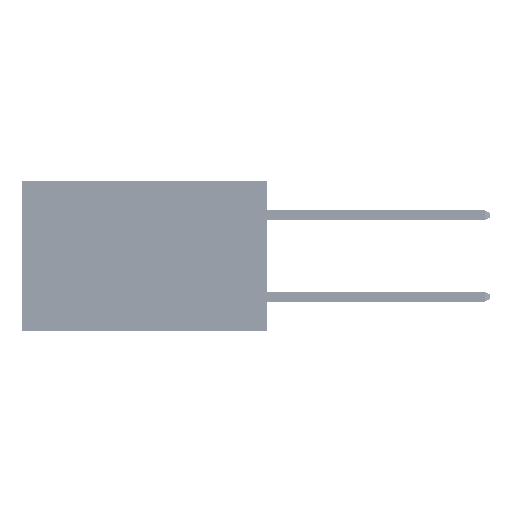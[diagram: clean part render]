
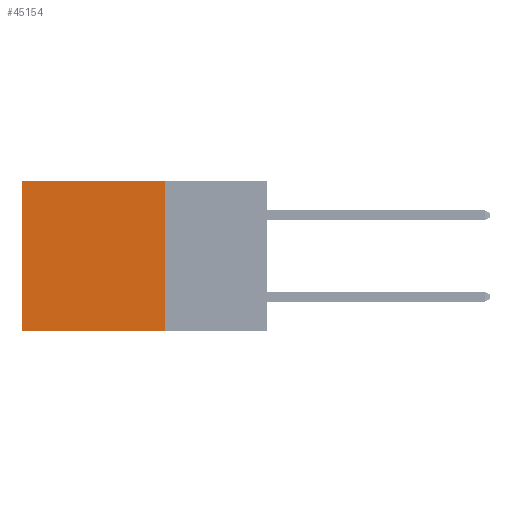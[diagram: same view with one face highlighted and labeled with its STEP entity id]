
A CAD part, left-side view. The second image highlights one B-rep face of the part: STEP entity #45154.
In plain terms, the highlighted planar face has unit normal (-1, 0, 0).
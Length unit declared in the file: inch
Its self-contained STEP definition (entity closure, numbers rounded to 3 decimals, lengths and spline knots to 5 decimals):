
#30 = VERTEX_POINT ( 'NONE', #20422 ) ;
#1703 = VECTOR ( 'NONE', #15579, 39.37008 ) ;
#3311 = EDGE_CURVE ( 'NONE', #30, #13991, #42936, .T. ) ;
#4253 = ORIENTED_EDGE ( 'NONE', *, *, #6570, .T. ) ;
#4584 = CARTESIAN_POINT ( 'NONE',  ( 0.2875, 0.25, 0. ) ) ;
#4908 = DIRECTION ( 'NONE',  ( 1., 0., 0. ) ) ;
#6570 = EDGE_CURVE ( 'NONE', #27314, #41171, #8188, .T. ) ;
#7189 = CARTESIAN_POINT ( 'NONE',  ( 0.2875, 0.25, -0.37 ) ) ;
#7624 = ORIENTED_EDGE ( 'NONE', *, *, #15448, .T. ) ;
#7821 = CARTESIAN_POINT ( 'NONE',  ( 0.2875, 0.6, 0. ) ) ;
#8188 = LINE ( 'NONE', #7821, #20060 ) ;
#9145 = AXIS2_PLACEMENT_3D ( 'NONE', #4584, #4908, #27328 ) ;
#9379 = FACE_OUTER_BOUND ( 'NONE', #45126, .T. ) ;
#10221 = CARTESIAN_POINT ( 'NONE',  ( 0.2875, 0.25, 0. ) ) ;
#10393 = VECTOR ( 'NONE', #16452, 39.37008 ) ;
#13991 = VERTEX_POINT ( 'NONE', #7189 ) ;
#15220 = CARTESIAN_POINT ( 'NONE',  ( 0.2875, 0.6, -0.37 ) ) ;
#15448 = EDGE_CURVE ( 'NONE', #30, #27314, #20520, .T. ) ;
#15579 = DIRECTION ( 'NONE',  ( 0., 1., 0. ) ) ;
#15879 = PLANE ( 'NONE',  #9145 ) ;
#16452 = DIRECTION ( 'NONE',  ( 0., 1., 0. ) ) ;
#19090 = CARTESIAN_POINT ( 'NONE',  ( 0.2875, 0.6, 0. ) ) ;
#20060 = VECTOR ( 'NONE', #33789, 39.37008 ) ;
#20422 = CARTESIAN_POINT ( 'NONE',  ( 0.2875, 0.25, 0. ) ) ;
#20520 = LINE ( 'NONE', #47054, #10393 ) ;
#22172 = DIRECTION ( 'NONE',  ( 0., 0., -1. ) ) ;
#25147 = EDGE_CURVE ( 'NONE', #13991, #41171, #33882, .T. ) ;
#27314 = VERTEX_POINT ( 'NONE', #19090 ) ;
#27328 = DIRECTION ( 'NONE',  ( 0., 0., -1. ) ) ;
#30229 = ORIENTED_EDGE ( 'NONE', *, *, #3311, .F. ) ;
#31370 = CARTESIAN_POINT ( 'NONE',  ( 0.2875, 0.25, -0.37 ) ) ;
#33329 = ORIENTED_EDGE ( 'NONE', *, *, #25147, .F. ) ;
#33789 = DIRECTION ( 'NONE',  ( 0., 0., -1. ) ) ;
#33882 = LINE ( 'NONE', #31370, #1703 ) ;
#35236 = VECTOR ( 'NONE', #22172, 39.37008 ) ;
#41171 = VERTEX_POINT ( 'NONE', #15220 ) ;
#42936 = LINE ( 'NONE', #10221, #35236 ) ;
#45126 = EDGE_LOOP ( 'NONE', ( #4253, #33329, #30229, #7624 ) ) ;
#45154 = ADVANCED_FACE ( 'NONE', ( #9379 ), #15879, .F. ) ;
#47054 = CARTESIAN_POINT ( 'NONE',  ( 0.2875, 0.25, 0. ) ) ;
